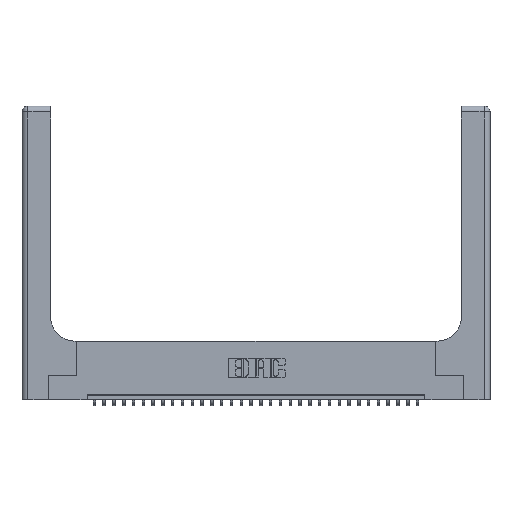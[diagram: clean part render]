
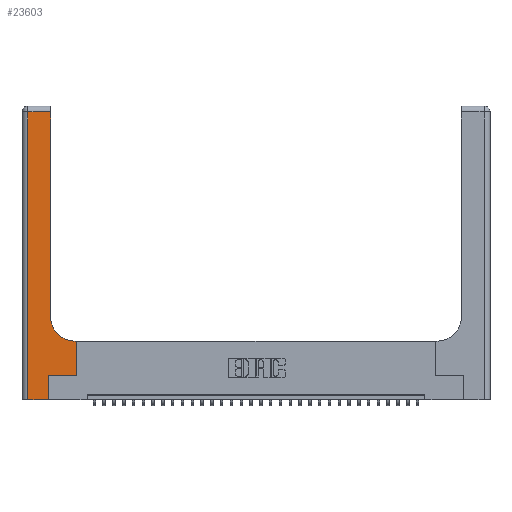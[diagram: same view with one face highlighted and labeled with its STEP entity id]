
A CAD part, top view. The second image highlights one B-rep face of the part: STEP entity #23603.
In plain terms, the highlighted planar face has unit normal (0, 0, 1).
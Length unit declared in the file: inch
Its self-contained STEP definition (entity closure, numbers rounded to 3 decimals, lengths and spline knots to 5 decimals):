
#384 = VECTOR ( 'NONE', #23928, 39.37008 ) ;
#1870 = ORIENTED_EDGE ( 'NONE', *, *, #29707, .T. ) ;
#1954 = VERTEX_POINT ( 'NONE', #28239 ) ;
#2526 = ORIENTED_EDGE ( 'NONE', *, *, #4943, .T. ) ;
#2624 = CARTESIAN_POINT ( 'NONE',  ( 0.2915, 3., 0.37 ) ) ;
#2639 = DIRECTION ( 'NONE',  ( -1., 0., 0. ) ) ;
#3739 = LINE ( 'NONE', #18575, #21125 ) ;
#3791 = ORIENTED_EDGE ( 'NONE', *, *, #28130, .T. ) ;
#4943 = EDGE_CURVE ( 'NONE', #19139, #27466, #29324, .T. ) ;
#5086 = EDGE_CURVE ( 'NONE', #16016, #1954, #21590, .T. ) ;
#5219 = LINE ( 'NONE', #2624, #30721 ) ;
#6135 = ORIENTED_EDGE ( 'NONE', *, *, #25087, .T. ) ;
#6235 = CARTESIAN_POINT ( 'NONE',  ( 0.06, 0., 0.37 ) ) ;
#8053 = ORIENTED_EDGE ( 'NONE', *, *, #25463, .T. ) ;
#8150 = CARTESIAN_POINT ( 'NONE',  ( 0., 0., 0.37 ) ) ;
#8683 = CARTESIAN_POINT ( 'NONE',  ( 0.5585, 0.25, 0.37 ) ) ;
#8826 = DIRECTION ( 'NONE',  ( 0., -1., 0. ) ) ;
#9205 = DIRECTION ( 'NONE',  ( 0., 0., -1. ) ) ;
#9833 = VERTEX_POINT ( 'NONE', #12492 ) ;
#10177 = LINE ( 'NONE', #31402, #15180 ) ;
#10200 = CARTESIAN_POINT ( 'NONE',  ( 0.5585, 0.6, 0.37 ) ) ;
#10271 = CARTESIAN_POINT ( 'NONE',  ( 0., 2.94, 0.37 ) ) ;
#10345 = DIRECTION ( 'NONE',  ( -1., 0., 0. ) ) ;
#10755 = VECTOR ( 'NONE', #29603, 39.37008 ) ;
#10934 = CARTESIAN_POINT ( 'NONE',  ( 0.5415, 0.6, 0.37 ) ) ;
#11770 = PLANE ( 'NONE',  #19443 ) ;
#12169 = VERTEX_POINT ( 'NONE', #10934 ) ;
#12315 = CARTESIAN_POINT ( 'NONE',  ( 0.269, 0., 0.37 ) ) ;
#12492 = CARTESIAN_POINT ( 'NONE',  ( 0.2915, 0.85, 0.37 ) ) ;
#12606 = CARTESIAN_POINT ( 'NONE',  ( 0.2915, 2.94, 0.37 ) ) ;
#13096 = LINE ( 'NONE', #8150, #17006 ) ;
#14358 = CARTESIAN_POINT ( 'NONE',  ( 0., 3., 0.37 ) ) ;
#15180 = VECTOR ( 'NONE', #28734, 39.37008 ) ;
#16016 = VERTEX_POINT ( 'NONE', #25744 ) ;
#16373 = CARTESIAN_POINT ( 'NONE',  ( 0.5585, 0.25, 0.37 ) ) ;
#17006 = VECTOR ( 'NONE', #30274, 39.37008 ) ;
#17498 = VECTOR ( 'NONE', #19272, 39.37008 ) ;
#17562 = CARTESIAN_POINT ( 'NONE',  ( 0.06, 2.94, 0.37 ) ) ;
#17565 = AXIS2_PLACEMENT_3D ( 'NONE', #26418, #9205, #23907 ) ;
#17692 = VERTEX_POINT ( 'NONE', #12606 ) ;
#18575 = CARTESIAN_POINT ( 'NONE',  ( 0.06, 3., 0.37 ) ) ;
#18922 = LINE ( 'NONE', #10271, #20832 ) ;
#19139 = VERTEX_POINT ( 'NONE', #8683 ) ;
#19272 = DIRECTION ( 'NONE',  ( 1., 0., 0. ) ) ;
#19443 = AXIS2_PLACEMENT_3D ( 'NONE', #14358, #28458, #10345 ) ;
#19461 = EDGE_CURVE ( 'NONE', #1954, #19139, #22530, .T. ) ;
#19560 = FACE_OUTER_BOUND ( 'NONE', #20747, .T. ) ;
#20669 = VERTEX_POINT ( 'NONE', #17562 ) ;
#20747 = EDGE_LOOP ( 'NONE', ( #1870, #3791, #22020, #28651, #30729, #24415, #2526, #8053, #6135 ) ) ;
#20832 = VECTOR ( 'NONE', #2639, 39.37008 ) ;
#21125 = VECTOR ( 'NONE', #8826, 39.37008 ) ;
#21198 = EDGE_CURVE ( 'NONE', #22483, #16016, #13096, .T. ) ;
#21590 = LINE ( 'NONE', #12315, #10755 ) ;
#22020 = ORIENTED_EDGE ( 'NONE', *, *, #22993, .T. ) ;
#22483 = VERTEX_POINT ( 'NONE', #6235 ) ;
#22530 = LINE ( 'NONE', #24574, #17498 ) ;
#22993 = EDGE_CURVE ( 'NONE', #20669, #22483, #3739, .T. ) ;
#23603 = ADVANCED_FACE ( 'NONE', ( #19560 ), #11770, .F. ) ;
#23907 = DIRECTION ( 'NONE',  ( 1., 0., 0. ) ) ;
#23928 = DIRECTION ( 'NONE',  ( 0., 1., 0. ) ) ;
#24415 = ORIENTED_EDGE ( 'NONE', *, *, #19461, .T. ) ;
#24574 = CARTESIAN_POINT ( 'NONE',  ( 0.269, 0.25, 0.37 ) ) ;
#25087 = EDGE_CURVE ( 'NONE', #12169, #9833, #30284, .T. ) ;
#25463 = EDGE_CURVE ( 'NONE', #27466, #12169, #10177, .T. ) ;
#25744 = CARTESIAN_POINT ( 'NONE',  ( 0.269, 0., 0.37 ) ) ;
#26418 = CARTESIAN_POINT ( 'NONE',  ( 0.5415, 0.85, 0.37 ) ) ;
#27466 = VERTEX_POINT ( 'NONE', #10200 ) ;
#28130 = EDGE_CURVE ( 'NONE', #17692, #20669, #18922, .T. ) ;
#28239 = CARTESIAN_POINT ( 'NONE',  ( 0.269, 0.25, 0.37 ) ) ;
#28458 = DIRECTION ( 'NONE',  ( 0., 0., -1. ) ) ;
#28651 = ORIENTED_EDGE ( 'NONE', *, *, #21198, .T. ) ;
#28734 = DIRECTION ( 'NONE',  ( -1., 0., 0. ) ) ;
#29324 = LINE ( 'NONE', #16373, #384 ) ;
#29491 = DIRECTION ( 'NONE',  ( 0., 1., 0. ) ) ;
#29603 = DIRECTION ( 'NONE',  ( 0., 1., 0. ) ) ;
#29707 = EDGE_CURVE ( 'NONE', #9833, #17692, #5219, .T. ) ;
#30274 = DIRECTION ( 'NONE',  ( 1., 0., 0. ) ) ;
#30284 = CIRCLE ( 'NONE', #17565, 0.25 ) ;
#30721 = VECTOR ( 'NONE', #29491, 39.37008 ) ;
#30729 = ORIENTED_EDGE ( 'NONE', *, *, #5086, .T. ) ;
#31402 = CARTESIAN_POINT ( 'NONE',  ( 0.2915, 0.6, 0.37 ) ) ;
